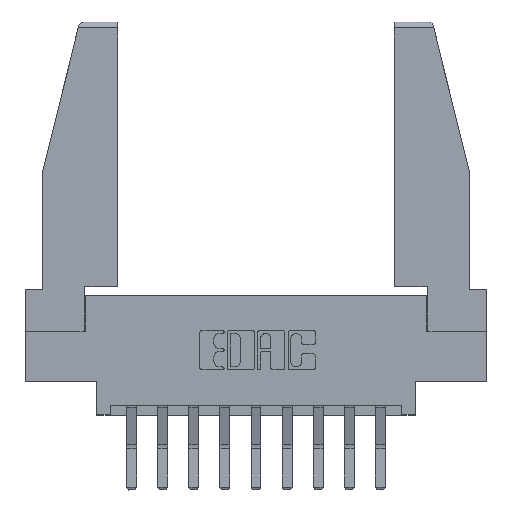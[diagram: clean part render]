
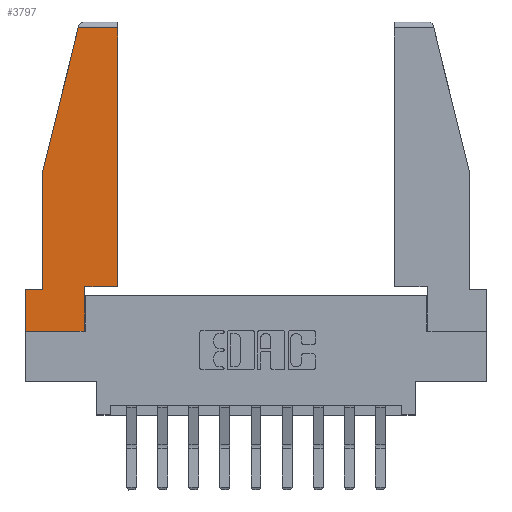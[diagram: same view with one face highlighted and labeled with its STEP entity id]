
A CAD part, top view. The second image highlights one B-rep face of the part: STEP entity #3797.
In plain terms, the highlighted planar face has unit normal (0, 0, 1).
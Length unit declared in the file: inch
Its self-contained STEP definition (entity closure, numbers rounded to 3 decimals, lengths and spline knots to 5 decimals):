
#105 = LINE ( 'NONE', #4037, #13217 ) ;
#114 = AXIS2_PLACEMENT_3D ( 'NONE', #4509, #7825, #8769 ) ;
#847 = CARTESIAN_POINT ( 'NONE',  ( 0.461, 1.52, 0. ) ) ;
#988 = DIRECTION ( 'NONE',  ( -1., 0., 0. ) ) ;
#1289 = LINE ( 'NONE', #2576, #9060 ) ;
#1455 = CARTESIAN_POINT ( 'NONE',  ( 0.297, 0., 0. ) ) ;
#1503 = ORIENTED_EDGE ( 'NONE', *, *, #6026, .T. ) ;
#1633 = LINE ( 'NONE', #9318, #9071 ) ;
#1681 = CARTESIAN_POINT ( 'NONE',  ( 0.461, 0.223, 0. ) ) ;
#1818 = VECTOR ( 'NONE', #7328, 39.37008 ) ;
#1987 = CARTESIAN_POINT ( 'NONE',  ( 0.086, 0.21, 0. ) ) ;
#2063 = PLANE ( 'NONE',  #114 ) ;
#2114 = LINE ( 'NONE', #11037, #12871 ) ;
#2141 = EDGE_CURVE ( 'NONE', #12349, #3550, #2114, .T. ) ;
#2576 = CARTESIAN_POINT ( 'NONE',  ( 0.461, 0.223, 0. ) ) ;
#2604 = VERTEX_POINT ( 'NONE', #5777 ) ;
#2697 = VERTEX_POINT ( 'NONE', #847 ) ;
#2735 = FACE_OUTER_BOUND ( 'NONE', #11165, .T. ) ;
#3115 = DIRECTION ( 'NONE',  ( 1., 0., 0. ) ) ;
#3248 = DIRECTION ( 'NONE',  ( 0., -1., 0. ) ) ;
#3550 = VERTEX_POINT ( 'NONE', #5683 ) ;
#3597 = LINE ( 'NONE', #10076, #4932 ) ;
#3633 = VERTEX_POINT ( 'NONE', #10452 ) ;
#3797 = ADVANCED_FACE ( 'NONE', ( #2735 ), #2063, .T. ) ;
#4037 = CARTESIAN_POINT ( 'NONE',  ( 0.297, 0.223, 0. ) ) ;
#4138 = VERTEX_POINT ( 'NONE', #8277 ) ;
#4337 = CARTESIAN_POINT ( 'NONE',  ( 0., 0.21, 0. ) ) ;
#4509 = CARTESIAN_POINT ( 'NONE',  ( 0., 0., 0. ) ) ;
#4565 = VERTEX_POINT ( 'NONE', #1681 ) ;
#4688 = DIRECTION ( 'NONE',  ( -1., 0., 0. ) ) ;
#4823 = ORIENTED_EDGE ( 'NONE', *, *, #6464, .T. ) ;
#4932 = VECTOR ( 'NONE', #4688, 39.37008 ) ;
#4978 = EDGE_CURVE ( 'NONE', #2604, #3633, #5360, .T. ) ;
#5081 = VECTOR ( 'NONE', #12131, 39.37008 ) ;
#5219 = EDGE_CURVE ( 'NONE', #3633, #9069, #6523, .T. ) ;
#5360 = LINE ( 'NONE', #11635, #1818 ) ;
#5453 = LINE ( 'NONE', #13773, #10325 ) ;
#5466 = LINE ( 'NONE', #1455, #5081 ) ;
#5683 = CARTESIAN_POINT ( 'NONE',  ( 0., 0., 0. ) ) ;
#5777 = CARTESIAN_POINT ( 'NONE',  ( 0.2636, 1.52, 0. ) ) ;
#6026 = EDGE_CURVE ( 'NONE', #9069, #12349, #1633, .T. ) ;
#6112 = ORIENTED_EDGE ( 'NONE', *, *, #2141, .T. ) ;
#6464 = EDGE_CURVE ( 'NONE', #13578, #4565, #105, .T. ) ;
#6523 = LINE ( 'NONE', #7300, #7029 ) ;
#6537 = ORIENTED_EDGE ( 'NONE', *, *, #10864, .T. ) ;
#6670 = EDGE_CURVE ( 'NONE', #4565, #2697, #1289, .T. ) ;
#6715 = CARTESIAN_POINT ( 'NONE',  ( 0.297, 0.223, 0. ) ) ;
#6855 = ORIENTED_EDGE ( 'NONE', *, *, #4978, .T. ) ;
#6906 = DIRECTION ( 'NONE',  ( 0., 1., 0. ) ) ;
#7013 = ORIENTED_EDGE ( 'NONE', *, *, #10185, .T. ) ;
#7029 = VECTOR ( 'NONE', #3248, 39.37008 ) ;
#7082 = EDGE_CURVE ( 'NONE', #2697, #2604, #3597, .T. ) ;
#7300 = CARTESIAN_POINT ( 'NONE',  ( 0.086, 0.8, 0. ) ) ;
#7328 = DIRECTION ( 'NONE',  ( -0.239, -0.971, 0. ) ) ;
#7825 = DIRECTION ( 'NONE',  ( 0., 0., 1. ) ) ;
#8277 = CARTESIAN_POINT ( 'NONE',  ( 0.297, 0., 0. ) ) ;
#8443 = ORIENTED_EDGE ( 'NONE', *, *, #5219, .T. ) ;
#8769 = DIRECTION ( 'NONE',  ( 1., 0., 0. ) ) ;
#9060 = VECTOR ( 'NONE', #6906, 39.37008 ) ;
#9069 = VERTEX_POINT ( 'NONE', #1987 ) ;
#9071 = VECTOR ( 'NONE', #988, 39.37008 ) ;
#9318 = CARTESIAN_POINT ( 'NONE',  ( 0., 0.21, 0. ) ) ;
#10076 = CARTESIAN_POINT ( 'NONE',  ( 0., 1.52, 0. ) ) ;
#10185 = EDGE_CURVE ( 'NONE', #4138, #13578, #5466, .T. ) ;
#10325 = VECTOR ( 'NONE', #3115, 39.37008 ) ;
#10403 = ORIENTED_EDGE ( 'NONE', *, *, #6670, .T. ) ;
#10452 = CARTESIAN_POINT ( 'NONE',  ( 0.086, 0.8, 0. ) ) ;
#10864 = EDGE_CURVE ( 'NONE', #3550, #4138, #5453, .T. ) ;
#10929 = ORIENTED_EDGE ( 'NONE', *, *, #7082, .T. ) ;
#10992 = DIRECTION ( 'NONE',  ( 0., -1., 0. ) ) ;
#11037 = CARTESIAN_POINT ( 'NONE',  ( 0., 0.21, 0. ) ) ;
#11165 = EDGE_LOOP ( 'NONE', ( #10403, #10929, #6855, #8443, #1503, #6112, #6537, #7013, #4823 ) ) ;
#11635 = CARTESIAN_POINT ( 'NONE',  ( 0.271, 1.55, 0. ) ) ;
#12131 = DIRECTION ( 'NONE',  ( 0., 1., 0. ) ) ;
#12349 = VERTEX_POINT ( 'NONE', #4337 ) ;
#12871 = VECTOR ( 'NONE', #10992, 39.37008 ) ;
#13217 = VECTOR ( 'NONE', #13623, 39.37008 ) ;
#13578 = VERTEX_POINT ( 'NONE', #6715 ) ;
#13623 = DIRECTION ( 'NONE',  ( 1., 0., 0. ) ) ;
#13773 = CARTESIAN_POINT ( 'NONE',  ( 0., 0., 0. ) ) ;
